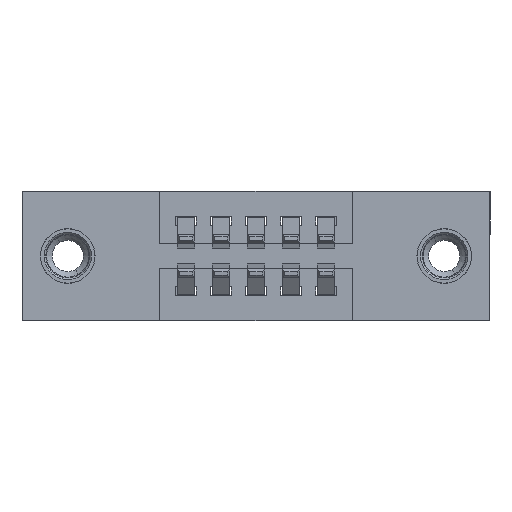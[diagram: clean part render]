
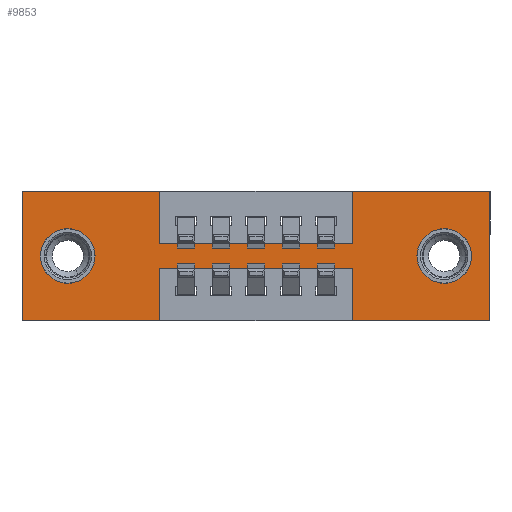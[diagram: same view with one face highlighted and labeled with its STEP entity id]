
A CAD part, front view. The second image highlights one B-rep face of the part: STEP entity #9853.
In plain terms, the highlighted planar face has unit normal (0, -1, 0).
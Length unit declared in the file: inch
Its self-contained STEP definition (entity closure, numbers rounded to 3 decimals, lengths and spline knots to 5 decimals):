
#16 = CARTESIAN_POINT ( 'NONE',  ( 0.13, 0., -0.185 ) ) ;
#19 = EDGE_CURVE ( 'NONE', #3176, #8598, #494, .T. ) ;
#141 = CARTESIAN_POINT ( 'NONE',  ( 1.335, 0., 0. ) ) ;
#185 = EDGE_CURVE ( 'NONE', #8797, #3310, #1708, .T. ) ;
#291 = ORIENTED_EDGE ( 'NONE', *, *, #12030, .F. ) ;
#392 = ORIENTED_EDGE ( 'NONE', *, *, #10254, .F. ) ;
#494 = LINE ( 'NONE', #5001, #11496 ) ;
#694 = EDGE_CURVE ( 'NONE', #9313, #11868, #4880, .T. ) ;
#841 = CARTESIAN_POINT ( 'NONE',  ( 0.13, 0., -0.185 ) ) ;
#1014 = LINE ( 'NONE', #9161, #11956 ) ;
#1053 = CARTESIAN_POINT ( 'NONE',  ( 0.3925, 0., -0.22 ) ) ;
#1159 = DIRECTION ( 'NONE',  ( 0., 0., 1. ) ) ;
#1231 = CARTESIAN_POINT ( 'NONE',  ( 1.335, 0., -0.37 ) ) ;
#1276 = DIRECTION ( 'NONE',  ( 0., 0., -1. ) ) ;
#1340 = VECTOR ( 'NONE', #1276, 39.37008 ) ;
#1495 = EDGE_LOOP ( 'NONE', ( #5852, #5188 ) ) ;
#1643 = DIRECTION ( 'NONE',  ( 0., 0., -1. ) ) ;
#1708 = LINE ( 'NONE', #9819, #5218 ) ;
#1709 = CARTESIAN_POINT ( 'NONE',  ( 1.335, 0., 0. ) ) ;
#1952 = DIRECTION ( 'NONE',  ( 0., 0., 1. ) ) ;
#2266 = EDGE_CURVE ( 'NONE', #3848, #12983, #13404, .T. ) ;
#2268 = EDGE_LOOP ( 'NONE', ( #291, #3093, #13272, #392, #3971, #2575, #6863, #9981, #5114, #10890, #10334, #13258 ) ) ;
#2291 = CARTESIAN_POINT ( 'NONE',  ( 0., 0., 0. ) ) ;
#2335 = LINE ( 'NONE', #8018, #2660 ) ;
#2411 = VERTEX_POINT ( 'NONE', #8409 ) ;
#2575 = ORIENTED_EDGE ( 'NONE', *, *, #19, .F. ) ;
#2631 = EDGE_CURVE ( 'NONE', #9803, #2411, #9854, .T. ) ;
#2660 = VECTOR ( 'NONE', #1643, 39.37008 ) ;
#2750 = DIRECTION ( 'NONE',  ( 0., 0., 1. ) ) ;
#2847 = CARTESIAN_POINT ( 'NONE',  ( 0.3925, 0., -0.15 ) ) ;
#3061 = AXIS2_PLACEMENT_3D ( 'NONE', #841, #8319, #1952 ) ;
#3093 = ORIENTED_EDGE ( 'NONE', *, *, #8188, .F. ) ;
#3176 = VERTEX_POINT ( 'NONE', #11198 ) ;
#3287 = CARTESIAN_POINT ( 'NONE',  ( 0.13, 0., -0.263 ) ) ;
#3310 = VERTEX_POINT ( 'NONE', #8255 ) ;
#3777 = VERTEX_POINT ( 'NONE', #3874 ) ;
#3822 = CARTESIAN_POINT ( 'NONE',  ( 0.9425, 0., 0. ) ) ;
#3848 = VERTEX_POINT ( 'NONE', #2847 ) ;
#3858 = EDGE_CURVE ( 'NONE', #6997, #3848, #9990, .T. ) ;
#3874 = CARTESIAN_POINT ( 'NONE',  ( 0.3925, 0., -0.37 ) ) ;
#3930 = CARTESIAN_POINT ( 'NONE',  ( 0., 0., -0.37 ) ) ;
#3971 = ORIENTED_EDGE ( 'NONE', *, *, #13752, .F. ) ;
#3991 = EDGE_CURVE ( 'NONE', #4916, #9416, #13523, .T. ) ;
#4138 = DIRECTION ( 'NONE',  ( 0., 0., 1. ) ) ;
#4215 = CARTESIAN_POINT ( 'NONE',  ( 0.9425, 0., -0.37 ) ) ;
#4221 = LINE ( 'NONE', #141, #1340 ) ;
#4392 = EDGE_CURVE ( 'NONE', #9416, #4916, #12045, .T. ) ;
#4586 = DIRECTION ( 'NONE',  ( 0., 0., 1. ) ) ;
#4608 = VERTEX_POINT ( 'NONE', #1231 ) ;
#4784 = LINE ( 'NONE', #2291, #9786 ) ;
#4880 = LINE ( 'NONE', #11790, #12614 ) ;
#4916 = VERTEX_POINT ( 'NONE', #7039 ) ;
#4936 = VECTOR ( 'NONE', #12400, 39.37008 ) ;
#5001 = CARTESIAN_POINT ( 'NONE',  ( 0., 0., 0. ) ) ;
#5073 = LINE ( 'NONE', #8201, #4936 ) ;
#5114 = ORIENTED_EDGE ( 'NONE', *, *, #3858, .F. ) ;
#5188 = ORIENTED_EDGE ( 'NONE', *, *, #4392, .T. ) ;
#5218 = VECTOR ( 'NONE', #4138, 39.37008 ) ;
#5545 = EDGE_CURVE ( 'NONE', #11868, #6997, #4784, .T. ) ;
#5652 = ORIENTED_EDGE ( 'NONE', *, *, #12703, .T. ) ;
#5839 = CARTESIAN_POINT ( 'NONE',  ( 1.205, 0., -0.185 ) ) ;
#5852 = ORIENTED_EDGE ( 'NONE', *, *, #3991, .T. ) ;
#5923 = CARTESIAN_POINT ( 'NONE',  ( 1.205, 0., -0.185 ) ) ;
#5939 = CARTESIAN_POINT ( 'NONE',  ( 0.3925, 0., 0. ) ) ;
#6183 = CARTESIAN_POINT ( 'NONE',  ( 0.3925, 0., -0.15 ) ) ;
#6249 = CARTESIAN_POINT ( 'NONE',  ( 0., 0., -0.37 ) ) ;
#6770 = AXIS2_PLACEMENT_3D ( 'NONE', #5923, #13285, #7003 ) ;
#6863 = ORIENTED_EDGE ( 'NONE', *, *, #12755, .F. ) ;
#6915 = DIRECTION ( 'NONE',  ( 0., 0., -1. ) ) ;
#6997 = VERTEX_POINT ( 'NONE', #5939 ) ;
#7003 = DIRECTION ( 'NONE',  ( 0., 0., -1. ) ) ;
#7039 = CARTESIAN_POINT ( 'NONE',  ( 0.13, 0., -0.107 ) ) ;
#7069 = PLANE ( 'NONE',  #8720 ) ;
#7114 = CARTESIAN_POINT ( 'NONE',  ( 0.3925, 0., 0. ) ) ;
#7116 = DIRECTION ( 'NONE',  ( 0., 0., -1. ) ) ;
#7541 = DIRECTION ( 'NONE',  ( 0., 1., 0. ) ) ;
#7572 = DIRECTION ( 'NONE',  ( 1., 0., 0. ) ) ;
#7857 = AXIS2_PLACEMENT_3D ( 'NONE', #16, #7541, #1159 ) ;
#8018 = CARTESIAN_POINT ( 'NONE',  ( 0.3925, 0., -0.37 ) ) ;
#8039 = VECTOR ( 'NONE', #2750, 39.37008 ) ;
#8058 = CARTESIAN_POINT ( 'NONE',  ( 1.205, 0., -0.107 ) ) ;
#8127 = EDGE_CURVE ( 'NONE', #3777, #9313, #5073, .T. ) ;
#8188 = EDGE_CURVE ( 'NONE', #3310, #8336, #9937, .T. ) ;
#8194 = DIRECTION ( 'NONE',  ( 0., 0., -1. ) ) ;
#8201 = CARTESIAN_POINT ( 'NONE',  ( 0., 0., -0.37 ) ) ;
#8211 = FACE_BOUND ( 'NONE', #1495, .T. ) ;
#8255 = CARTESIAN_POINT ( 'NONE',  ( 0.9425, 0., -0.22 ) ) ;
#8319 = DIRECTION ( 'NONE',  ( 0., 1., 0. ) ) ;
#8336 = VERTEX_POINT ( 'NONE', #1053 ) ;
#8359 = DIRECTION ( 'NONE',  ( 1., 0., 0. ) ) ;
#8409 = CARTESIAN_POINT ( 'NONE',  ( 1.205, 0., -0.263 ) ) ;
#8532 = DIRECTION ( 'NONE',  ( 1., 0., 0. ) ) ;
#8598 = VERTEX_POINT ( 'NONE', #1709 ) ;
#8720 = AXIS2_PLACEMENT_3D ( 'NONE', #3930, #13396, #7116 ) ;
#8723 = CARTESIAN_POINT ( 'NONE',  ( 0., 0., 0. ) ) ;
#8797 = VERTEX_POINT ( 'NONE', #4215 ) ;
#9161 = CARTESIAN_POINT ( 'NONE',  ( 0., 0., -0.37 ) ) ;
#9313 = VERTEX_POINT ( 'NONE', #6249 ) ;
#9320 = ORIENTED_EDGE ( 'NONE', *, *, #2631, .T. ) ;
#9416 = VERTEX_POINT ( 'NONE', #3287 ) ;
#9786 = VECTOR ( 'NONE', #7572, 39.37008 ) ;
#9803 = VERTEX_POINT ( 'NONE', #8058 ) ;
#9819 = CARTESIAN_POINT ( 'NONE',  ( 0.9425, 0., -0.37 ) ) ;
#9853 = ADVANCED_FACE ( 'NONE', ( #13762, #8211, #13433 ), #7069, .T. ) ;
#9854 = CIRCLE ( 'NONE', #6770, 0.078 ) ;
#9918 = AXIS2_PLACEMENT_3D ( 'NONE', #5839, #13204, #6915 ) ;
#9937 = LINE ( 'NONE', #12486, #12675 ) ;
#9981 = ORIENTED_EDGE ( 'NONE', *, *, #2266, .F. ) ;
#9990 = LINE ( 'NONE', #7114, #12058 ) ;
#10238 = DIRECTION ( 'NONE',  ( -1., 0., 0. ) ) ;
#10254 = EDGE_CURVE ( 'NONE', #4608, #8797, #1014, .T. ) ;
#10334 = ORIENTED_EDGE ( 'NONE', *, *, #694, .F. ) ;
#10342 = VECTOR ( 'NONE', #8532, 39.37008 ) ;
#10602 = CARTESIAN_POINT ( 'NONE',  ( 0.9425, 0., -0.15 ) ) ;
#10890 = ORIENTED_EDGE ( 'NONE', *, *, #5545, .F. ) ;
#11198 = CARTESIAN_POINT ( 'NONE',  ( 0.9425, 0., 0. ) ) ;
#11493 = CIRCLE ( 'NONE', #9918, 0.078 ) ;
#11496 = VECTOR ( 'NONE', #8359, 39.37008 ) ;
#11790 = CARTESIAN_POINT ( 'NONE',  ( 0., 0., 0. ) ) ;
#11868 = VERTEX_POINT ( 'NONE', #8723 ) ;
#11956 = VECTOR ( 'NONE', #10238, 39.37008 ) ;
#12030 = EDGE_CURVE ( 'NONE', #8336, #3777, #2335, .T. ) ;
#12045 = CIRCLE ( 'NONE', #3061, 0.078 ) ;
#12058 = VECTOR ( 'NONE', #8194, 39.37008 ) ;
#12400 = DIRECTION ( 'NONE',  ( -1., 0., 0. ) ) ;
#12486 = CARTESIAN_POINT ( 'NONE',  ( 0.3925, 0., -0.22 ) ) ;
#12614 = VECTOR ( 'NONE', #4586, 39.37008 ) ;
#12675 = VECTOR ( 'NONE', #13535, 39.37008 ) ;
#12703 = EDGE_CURVE ( 'NONE', #2411, #9803, #11493, .T. ) ;
#12755 = EDGE_CURVE ( 'NONE', #12983, #3176, #13259, .T. ) ;
#12983 = VERTEX_POINT ( 'NONE', #10602 ) ;
#13204 = DIRECTION ( 'NONE',  ( 0., 1., 0. ) ) ;
#13258 = ORIENTED_EDGE ( 'NONE', *, *, #8127, .F. ) ;
#13259 = LINE ( 'NONE', #3822, #8039 ) ;
#13272 = ORIENTED_EDGE ( 'NONE', *, *, #185, .F. ) ;
#13285 = DIRECTION ( 'NONE',  ( 0., 1., 0. ) ) ;
#13396 = DIRECTION ( 'NONE',  ( 0., -1., 0. ) ) ;
#13404 = LINE ( 'NONE', #6183, #10342 ) ;
#13433 = FACE_OUTER_BOUND ( 'NONE', #2268, .T. ) ;
#13523 = CIRCLE ( 'NONE', #7857, 0.078 ) ;
#13535 = DIRECTION ( 'NONE',  ( -1., 0., 0. ) ) ;
#13639 = EDGE_LOOP ( 'NONE', ( #9320, #5652 ) ) ;
#13752 = EDGE_CURVE ( 'NONE', #8598, #4608, #4221, .T. ) ;
#13762 = FACE_BOUND ( 'NONE', #13639, .T. ) ;
